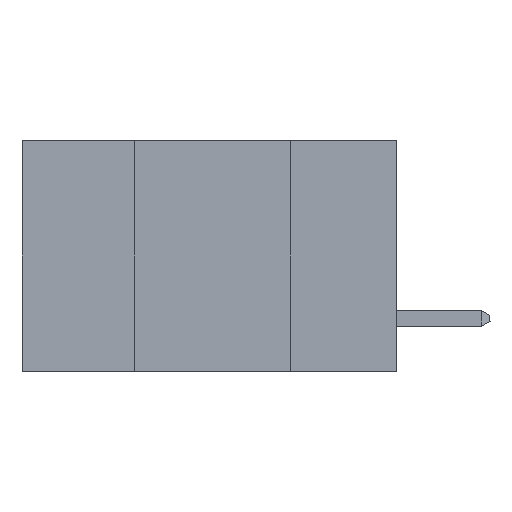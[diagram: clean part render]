
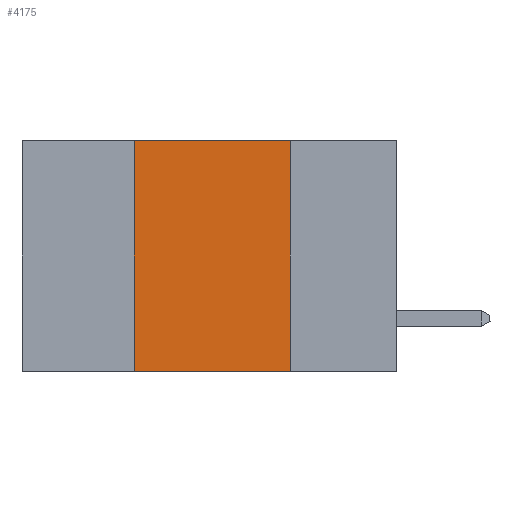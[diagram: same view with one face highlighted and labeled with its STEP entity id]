
A CAD part, left-side view. The second image highlights one B-rep face of the part: STEP entity #4175.
In plain terms, the highlighted planar face has unit normal (-1, 0, 0).
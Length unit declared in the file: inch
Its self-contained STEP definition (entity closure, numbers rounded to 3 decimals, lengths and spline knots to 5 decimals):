
#55 = ORIENTED_EDGE ( 'NONE', *, *, #12933, .F. ) ;
#68 = EDGE_CURVE ( 'NONE', #571, #3527, #12293, .T. ) ;
#139 = CARTESIAN_POINT ( 'NONE',  ( 0., 0.6, -0.37 ) ) ;
#571 = VERTEX_POINT ( 'NONE', #5222 ) ;
#714 = CARTESIAN_POINT ( 'NONE',  ( 0., 0.42, 0. ) ) ;
#766 = DIRECTION ( 'NONE',  ( 0., 0., 1. ) ) ;
#1260 = DIRECTION ( 'NONE',  ( 0., -1., 0. ) ) ;
#2016 = DIRECTION ( 'NONE',  ( 0., 0., -1. ) ) ;
#2024 = DIRECTION ( 'NONE',  ( 1., 0., 0. ) ) ;
#2167 = CARTESIAN_POINT ( 'NONE',  ( 0., 0.6, 0. ) ) ;
#2265 = PLANE ( 'NONE',  #4300 ) ;
#2288 = EDGE_CURVE ( 'NONE', #4652, #5425, #7580, .T. ) ;
#3387 = VECTOR ( 'NONE', #766, 39.37008 ) ;
#3527 = VERTEX_POINT ( 'NONE', #16081 ) ;
#4091 = EDGE_LOOP ( 'NONE', ( #55, #11138, #13151, #6707 ) ) ;
#4130 = VECTOR ( 'NONE', #1260, 39.37008 ) ;
#4175 = ADVANCED_FACE ( 'NONE', ( #11766 ), #2265, .F. ) ;
#4300 = AXIS2_PLACEMENT_3D ( 'NONE', #2167, #2024, #2016 ) ;
#4652 = VERTEX_POINT ( 'NONE', #14249 ) ;
#5222 = CARTESIAN_POINT ( 'NONE',  ( 0., 0.42, -0.37 ) ) ;
#5425 = VERTEX_POINT ( 'NONE', #8169 ) ;
#6707 = ORIENTED_EDGE ( 'NONE', *, *, #68, .T. ) ;
#7334 = CARTESIAN_POINT ( 'NONE',  ( 0., 0.17, 0. ) ) ;
#7580 = LINE ( 'NONE', #13873, #4130 ) ;
#8097 = VECTOR ( 'NONE', #8620, 39.37008 ) ;
#8169 = CARTESIAN_POINT ( 'NONE',  ( 0., 0.17, 0. ) ) ;
#8473 = VECTOR ( 'NONE', #13634, 39.37008 ) ;
#8620 = DIRECTION ( 'NONE',  ( 0., 0., -1. ) ) ;
#11138 = ORIENTED_EDGE ( 'NONE', *, *, #2288, .F. ) ;
#11508 = LINE ( 'NONE', #7334, #8097 ) ;
#11766 = FACE_OUTER_BOUND ( 'NONE', #4091, .T. ) ;
#12293 = LINE ( 'NONE', #139, #8473 ) ;
#12933 = EDGE_CURVE ( 'NONE', #5425, #3527, #11508, .T. ) ;
#13151 = ORIENTED_EDGE ( 'NONE', *, *, #14312, .F. ) ;
#13634 = DIRECTION ( 'NONE',  ( 0., -1., 0. ) ) ;
#13665 = LINE ( 'NONE', #714, #3387 ) ;
#13873 = CARTESIAN_POINT ( 'NONE',  ( 0., 0.6, 0. ) ) ;
#14249 = CARTESIAN_POINT ( 'NONE',  ( 0., 0.42, 0. ) ) ;
#14312 = EDGE_CURVE ( 'NONE', #571, #4652, #13665, .T. ) ;
#16081 = CARTESIAN_POINT ( 'NONE',  ( 0., 0.17, -0.37 ) ) ;
